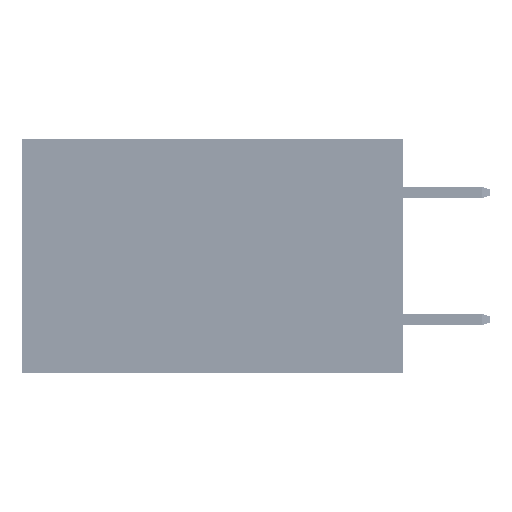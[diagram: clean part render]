
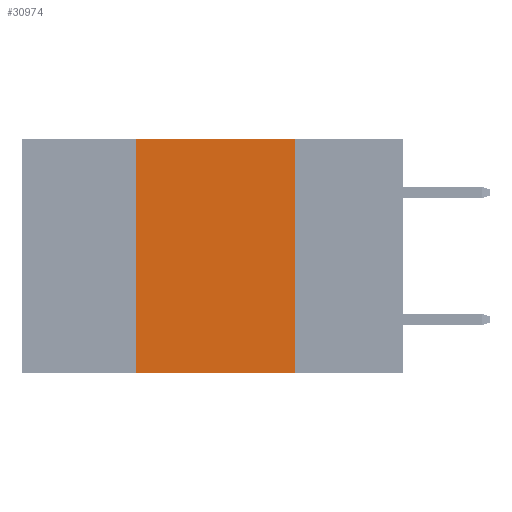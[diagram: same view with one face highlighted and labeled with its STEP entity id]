
A CAD part, left-side view. The second image highlights one B-rep face of the part: STEP entity #30974.
In plain terms, the highlighted planar face has unit normal (-1, 0, 0).
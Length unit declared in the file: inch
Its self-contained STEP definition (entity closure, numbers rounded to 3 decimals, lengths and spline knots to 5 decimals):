
#253 = EDGE_CURVE ( 'NONE', #31995, #4941, #21361, .T. ) ;
#671 = PLANE ( 'NONE',  #37599 ) ;
#1614 = EDGE_CURVE ( 'NONE', #21460, #31995, #5125, .T. ) ;
#1684 = CARTESIAN_POINT ( 'NONE',  ( 0., 0.42, 0. ) ) ;
#4339 = CARTESIAN_POINT ( 'NONE',  ( 0., 0.6, 0. ) ) ;
#4941 = VERTEX_POINT ( 'NONE', #11086 ) ;
#5125 = LINE ( 'NONE', #39897, #16078 ) ;
#5306 = DIRECTION ( 'NONE',  ( 0., 0., -1. ) ) ;
#7602 = VERTEX_POINT ( 'NONE', #29116 ) ;
#10503 = DIRECTION ( 'NONE',  ( 0., -1., 0. ) ) ;
#11086 = CARTESIAN_POINT ( 'NONE',  ( 0., 0.17, 0. ) ) ;
#11432 = VECTOR ( 'NONE', #34151, 39.37008 ) ;
#11690 = CARTESIAN_POINT ( 'NONE',  ( 0., 0.42, -0.37 ) ) ;
#15731 = DIRECTION ( 'NONE',  ( 1., 0., 0. ) ) ;
#16078 = VECTOR ( 'NONE', #35966, 39.37008 ) ;
#21361 = LINE ( 'NONE', #35893, #29491 ) ;
#21460 = VERTEX_POINT ( 'NONE', #11690 ) ;
#25024 = ORIENTED_EDGE ( 'NONE', *, *, #253, .F. ) ;
#26283 = CARTESIAN_POINT ( 'NONE',  ( 0., 0.6, -0.37 ) ) ;
#29116 = CARTESIAN_POINT ( 'NONE',  ( 0., 0.17, -0.37 ) ) ;
#29491 = VECTOR ( 'NONE', #10503, 39.37008 ) ;
#30222 = ORIENTED_EDGE ( 'NONE', *, *, #43420, .T. ) ;
#30757 = DIRECTION ( 'NONE',  ( 0., 0., -1. ) ) ;
#30974 = ADVANCED_FACE ( 'NONE', ( #38117 ), #671, .F. ) ;
#31943 = VECTOR ( 'NONE', #5306, 39.37008 ) ;
#31995 = VERTEX_POINT ( 'NONE', #1684 ) ;
#34151 = DIRECTION ( 'NONE',  ( 0., -1., 0. ) ) ;
#35893 = CARTESIAN_POINT ( 'NONE',  ( 0., 0.6, 0. ) ) ;
#35966 = DIRECTION ( 'NONE',  ( 0., 0., 1. ) ) ;
#36691 = ORIENTED_EDGE ( 'NONE', *, *, #1614, .F. ) ;
#37599 = AXIS2_PLACEMENT_3D ( 'NONE', #4339, #15731, #30757 ) ;
#37834 = LINE ( 'NONE', #26283, #11432 ) ;
#38117 = FACE_OUTER_BOUND ( 'NONE', #39929, .T. ) ;
#39091 = CARTESIAN_POINT ( 'NONE',  ( 0., 0.17, 0. ) ) ;
#39462 = ORIENTED_EDGE ( 'NONE', *, *, #40771, .F. ) ;
#39897 = CARTESIAN_POINT ( 'NONE',  ( 0., 0.42, 0. ) ) ;
#39929 = EDGE_LOOP ( 'NONE', ( #39462, #25024, #36691, #30222 ) ) ;
#40771 = EDGE_CURVE ( 'NONE', #4941, #7602, #42068, .T. ) ;
#42068 = LINE ( 'NONE', #39091, #31943 ) ;
#43420 = EDGE_CURVE ( 'NONE', #21460, #7602, #37834, .T. ) ;
